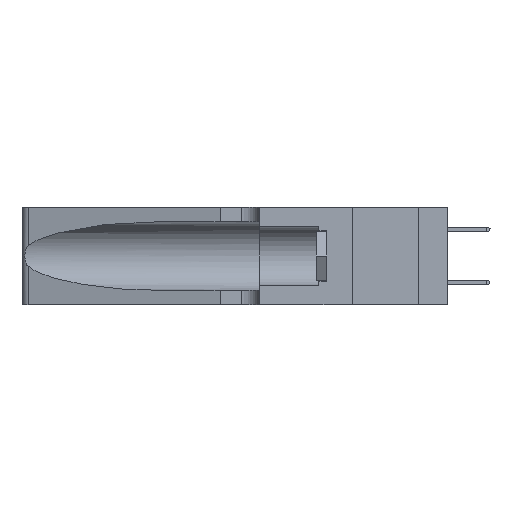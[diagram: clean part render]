
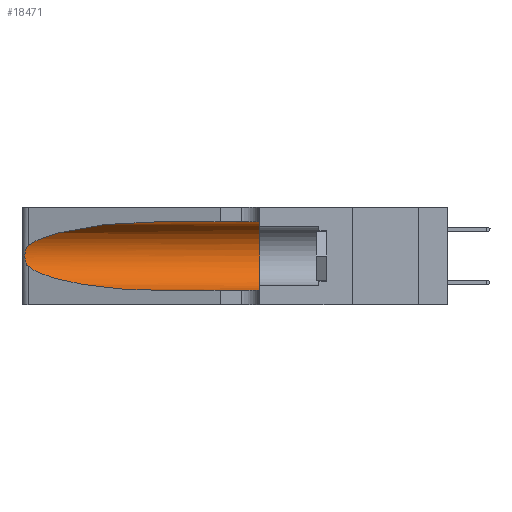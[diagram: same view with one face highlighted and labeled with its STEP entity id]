
A CAD part, left-side view. The second image highlights one B-rep face of the part: STEP entity #18471.
In plain terms, the highlighted cylindrical face has radius 3.308 mm (diameter 6.617 mm), a partial arc.
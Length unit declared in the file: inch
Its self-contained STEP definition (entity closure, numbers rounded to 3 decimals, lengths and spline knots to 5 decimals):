
#1313 = AXIS2_PLACEMENT_3D ( 'NONE', #16725, #2007, #19144 ) ;
#1842 = CARTESIAN_POINT ( 'NONE',  ( 0.26017, 1.23833, 0.17102 ) ) ;
#1927 = B_SPLINE_CURVE_WITH_KNOTS ( 'NONE', 3,
 ( #9145, #16448, #26000, #11689, #28409, #14115, #30816, #16571, #1842, #18985, #4377, #21361, #6876, #23760 ),
 .UNSPECIFIED., .F., .F.,
 ( 4, 2, 2, 2, 2, 2, 4 ),
 ( 0., 0.00027, 0.00053, 0.00107, 0.0016, 0.00187, 0.00214 ),
 .UNSPECIFIED. ) ;
#2007 = DIRECTION ( 'NONE',  ( 0., 1., 0. ) ) ;
#2178 = CARTESIAN_POINT ( 'NONE',  ( 0.25487, 1.22718, 0.14631 ) ) ;
#2680 = DIRECTION ( 'NONE',  ( 0., 0., -1. ) ) ;
#3920 = CARTESIAN_POINT ( 'NONE',  ( 0.25487, 1.22718, 0.22369 ) ) ;
#4354 = VERTEX_POINT ( 'NONE', #29160 ) ;
#4377 = CARTESIAN_POINT ( 'NONE',  ( 0.25789, 1.23486, 0.15765 ) ) ;
#5517 = CIRCLE ( 'NONE', #1313, 0.13025 ) ;
#6876 = CARTESIAN_POINT ( 'NONE',  ( 0.25555, 1.22993, 0.14849 ) ) ;
#7372 = AXIS2_PLACEMENT_3D ( 'NONE', #7715, #10172, #2680 ) ;
#7715 = CARTESIAN_POINT ( 'NONE',  ( 0.1305, 1.61858, 0.185 ) ) ;
#7810 = ORIENTED_EDGE ( 'NONE', *, *, #26688, .T. ) ;
#8074 = CARTESIAN_POINT ( 'NONE',  ( 0.2373, 1.15595, 0.08982 ) ) ;
#8180 = CARTESIAN_POINT ( 'NONE',  ( 0.18966, 0.96281, 0.05475 ) ) ;
#9145 = CARTESIAN_POINT ( 'NONE',  ( 0.25487, 1.22718, 0.22369 ) ) ;
#10084 =( BOUNDED_CURVE ( )  B_SPLINE_CURVE ( 3, ( #30370, #16111, #18555, #3920 ),
 .UNSPECIFIED., .F., .F. ) 
 B_SPLINE_CURVE_WITH_KNOTS ( ( 4, 4 ),
 ( 1.5708, 2.84003 ),
 .UNSPECIFIED. ) 
 CURVE ( )  GEOMETRIC_REPRESENTATION_ITEM ( )  RATIONAL_B_SPLINE_CURVE ( ( 1., 0.87, 0.87, 1. ) ) 
 REPRESENTATION_ITEM ( '' )  );
#10172 = DIRECTION ( 'NONE',  ( 0., -1., 0. ) ) ;
#10432 = LINE ( 'NONE', #23827, #22459 ) ;
#11689 = CARTESIAN_POINT ( 'NONE',  ( 0.25787, 1.23484, 0.2124 ) ) ;
#12381 = EDGE_CURVE ( 'NONE', #4354, #29753, #10084, .T. ) ;
#13040 = FACE_OUTER_BOUND ( 'NONE', #15896, .T. ) ;
#13064 = CARTESIAN_POINT ( 'NONE',  ( 0.25487, 1.22718, 0.14631 ) ) ;
#14071 = CARTESIAN_POINT ( 'NONE',  ( 0.1305, 1.61858, 0.31525 ) ) ;
#14115 = CARTESIAN_POINT ( 'NONE',  ( 0.26018, 1.23835, 0.19895 ) ) ;
#14230 = EDGE_CURVE ( 'NONE', #19701, #23432, #30028, .T. ) ;
#14732 = VERTEX_POINT ( 'NONE', #29116 ) ;
#15474 = CARTESIAN_POINT ( 'NONE',  ( 0.1305, 0.72297, 0.05475 ) ) ;
#15896 = EDGE_LOOP ( 'NONE', ( #29611, #7810, #17049, #29059, #31278, #18349 ) ) ;
#16111 = CARTESIAN_POINT ( 'NONE',  ( 0.18966, 0.96281, 0.31525 ) ) ;
#16424 = VECTOR ( 'NONE', #16521, 39.37008 ) ;
#16448 = CARTESIAN_POINT ( 'NONE',  ( 0.25555, 1.22994, 0.2215 ) ) ;
#16521 = DIRECTION ( 'NONE',  ( 0., -1., 0. ) ) ;
#16571 = CARTESIAN_POINT ( 'NONE',  ( 0.26075, 1.23896, 0.178 ) ) ;
#16725 = CARTESIAN_POINT ( 'NONE',  ( 0.1305, 0.35, 0.185 ) ) ;
#17049 = ORIENTED_EDGE ( 'NONE', *, *, #14230, .T. ) ;
#18349 = ORIENTED_EDGE ( 'NONE', *, *, #28877, .F. ) ;
#18471 = ADVANCED_FACE ( 'NONE', ( #13040 ), #25009, .F. ) ;
#18555 = CARTESIAN_POINT ( 'NONE',  ( 0.2373, 1.15595, 0.28018 ) ) ;
#18985 = CARTESIAN_POINT ( 'NONE',  ( 0.25856, 1.23593, 0.16098 ) ) ;
#19144 = DIRECTION ( 'NONE',  ( 0., 0., 1. ) ) ;
#19518 = CARTESIAN_POINT ( 'NONE',  ( 0.25487, 1.22718, 0.22369 ) ) ;
#19701 = VERTEX_POINT ( 'NONE', #2178 ) ;
#20215 = CARTESIAN_POINT ( 'NONE',  ( 0.1305, 0.72297, 0.05475 ) ) ;
#20810 = EDGE_CURVE ( 'NONE', #14732, #23120, #5517, .T. ) ;
#21361 = CARTESIAN_POINT ( 'NONE',  ( 0.25639, 1.23186, 0.15144 ) ) ;
#21477 = CARTESIAN_POINT ( 'NONE',  ( 0.1305, 0.35, 0.05475 ) ) ;
#21936 = EDGE_CURVE ( 'NONE', #23432, #23120, #10432, .T. ) ;
#22459 = VECTOR ( 'NONE', #26168, 39.37008 ) ;
#22778 = LINE ( 'NONE', #14071, #16424 ) ;
#23120 = VERTEX_POINT ( 'NONE', #21477 ) ;
#23432 = VERTEX_POINT ( 'NONE', #20215 ) ;
#23760 = CARTESIAN_POINT ( 'NONE',  ( 0.25487, 1.22718, 0.14631 ) ) ;
#23827 = CARTESIAN_POINT ( 'NONE',  ( 0.1305, 1.61858, 0.05475 ) ) ;
#25009 = CYLINDRICAL_SURFACE ( 'NONE', #7372, 0.13025 ) ;
#26000 = CARTESIAN_POINT ( 'NONE',  ( 0.25639, 1.23184, 0.21858 ) ) ;
#26168 = DIRECTION ( 'NONE',  ( 0., -1., 0. ) ) ;
#26688 = EDGE_CURVE ( 'NONE', #29753, #19701, #1927, .T. ) ;
#28409 = CARTESIAN_POINT ( 'NONE',  ( 0.25854, 1.2359, 0.20912 ) ) ;
#28877 = EDGE_CURVE ( 'NONE', #4354, #14732, #22778, .T. ) ;
#29059 = ORIENTED_EDGE ( 'NONE', *, *, #21936, .T. ) ;
#29116 = CARTESIAN_POINT ( 'NONE',  ( 0.1305, 0.35, 0.31525 ) ) ;
#29160 = CARTESIAN_POINT ( 'NONE',  ( 0.1305, 0.72297, 0.31525 ) ) ;
#29611 = ORIENTED_EDGE ( 'NONE', *, *, #12381, .T. ) ;
#29753 = VERTEX_POINT ( 'NONE', #19518 ) ;
#30028 =( BOUNDED_CURVE ( )  B_SPLINE_CURVE ( 3, ( #13064, #8074, #8180, #15474 ),
 .UNSPECIFIED., .F., .F. ) 
 B_SPLINE_CURVE_WITH_KNOTS ( ( 4, 4 ),
 ( 3.44316, 4.71239 ),
 .UNSPECIFIED. ) 
 CURVE ( )  GEOMETRIC_REPRESENTATION_ITEM ( )  RATIONAL_B_SPLINE_CURVE ( ( 1., 0.87, 0.87, 1. ) ) 
 REPRESENTATION_ITEM ( '' )  );
#30370 = CARTESIAN_POINT ( 'NONE',  ( 0.1305, 0.72297, 0.31525 ) ) ;
#30816 = CARTESIAN_POINT ( 'NONE',  ( 0.26075, 1.23896, 0.19203 ) ) ;
#31278 = ORIENTED_EDGE ( 'NONE', *, *, #20810, .F. ) ;
